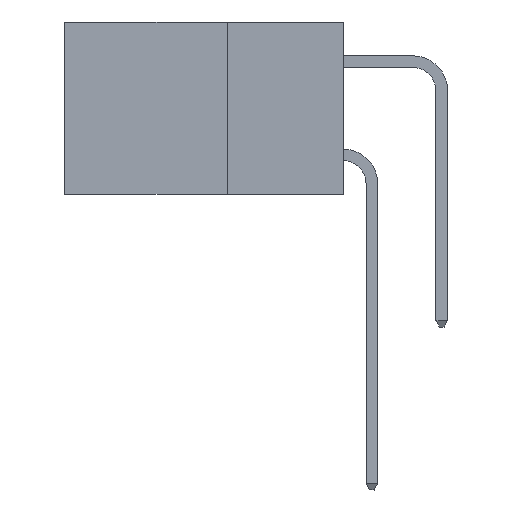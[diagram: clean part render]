
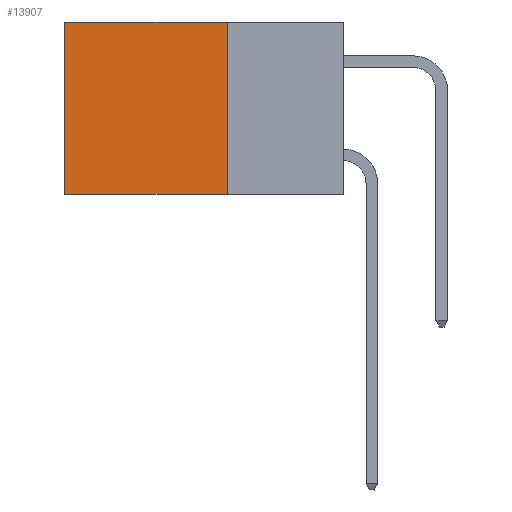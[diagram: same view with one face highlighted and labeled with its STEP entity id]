
A CAD part, left-side view. The second image highlights one B-rep face of the part: STEP entity #13907.
In plain terms, the highlighted planar face has unit normal (-1, 0, 0).
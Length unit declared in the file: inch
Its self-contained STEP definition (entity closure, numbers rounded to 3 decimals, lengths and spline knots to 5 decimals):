
#242 = VERTEX_POINT ( 'NONE', #3042 ) ;
#254 = FACE_OUTER_BOUND ( 'NONE', #14328, .T. ) ;
#332 = CARTESIAN_POINT ( 'NONE',  ( 0.298, 0.25, 0. ) ) ;
#626 = VECTOR ( 'NONE', #5358, 39.37008 ) ;
#683 = VERTEX_POINT ( 'NONE', #4844 ) ;
#1060 = LINE ( 'NONE', #13029, #12793 ) ;
#1148 = VERTEX_POINT ( 'NONE', #13455 ) ;
#2207 = ORIENTED_EDGE ( 'NONE', *, *, #9824, .T. ) ;
#3042 = CARTESIAN_POINT ( 'NONE',  ( 0.298, 0.6, -0.37 ) ) ;
#3738 = LINE ( 'NONE', #5139, #11578 ) ;
#3931 = CARTESIAN_POINT ( 'NONE',  ( 0.298, 0.25, 0. ) ) ;
#4036 = DIRECTION ( 'NONE',  ( 0., 0., -1. ) ) ;
#4844 = CARTESIAN_POINT ( 'NONE',  ( 0.298, 0.6, 0. ) ) ;
#5139 = CARTESIAN_POINT ( 'NONE',  ( 0.298, 0.25, 0. ) ) ;
#5358 = DIRECTION ( 'NONE',  ( 0., 1., 0. ) ) ;
#5772 = EDGE_CURVE ( 'NONE', #1148, #242, #1060, .T. ) ;
#6038 = EDGE_CURVE ( 'NONE', #683, #242, #7303, .T. ) ;
#6498 = DIRECTION ( 'NONE',  ( 0., 0., -1. ) ) ;
#6669 = VERTEX_POINT ( 'NONE', #8089 ) ;
#7112 = EDGE_CURVE ( 'NONE', #6669, #1148, #3738, .T. ) ;
#7303 = LINE ( 'NONE', #16142, #11436 ) ;
#8089 = CARTESIAN_POINT ( 'NONE',  ( 0.298, 0.25, 0. ) ) ;
#8652 = DIRECTION ( 'NONE',  ( 0., 0., -1. ) ) ;
#9775 = LINE ( 'NONE', #332, #626 ) ;
#9824 = EDGE_CURVE ( 'NONE', #6669, #683, #9775, .T. ) ;
#10146 = DIRECTION ( 'NONE',  ( 1., 0., 0. ) ) ;
#10392 = ORIENTED_EDGE ( 'NONE', *, *, #7112, .F. ) ;
#10647 = AXIS2_PLACEMENT_3D ( 'NONE', #3931, #10146, #6498 ) ;
#11436 = VECTOR ( 'NONE', #8652, 39.37008 ) ;
#11578 = VECTOR ( 'NONE', #4036, 39.37008 ) ;
#12793 = VECTOR ( 'NONE', #14379, 39.37008 ) ;
#13029 = CARTESIAN_POINT ( 'NONE',  ( 0.298, 0.25, -0.37 ) ) ;
#13455 = CARTESIAN_POINT ( 'NONE',  ( 0.298, 0.25, -0.37 ) ) ;
#13735 = ORIENTED_EDGE ( 'NONE', *, *, #6038, .T. ) ;
#13907 = ADVANCED_FACE ( 'NONE', ( #254 ), #15240, .F. ) ;
#14328 = EDGE_LOOP ( 'NONE', ( #13735, #16094, #10392, #2207 ) ) ;
#14379 = DIRECTION ( 'NONE',  ( 0., 1., 0. ) ) ;
#15240 = PLANE ( 'NONE',  #10647 ) ;
#16094 = ORIENTED_EDGE ( 'NONE', *, *, #5772, .F. ) ;
#16142 = CARTESIAN_POINT ( 'NONE',  ( 0.298, 0.6, 0. ) ) ;
